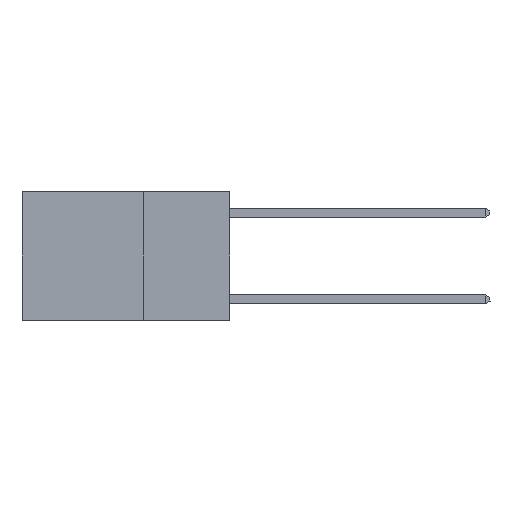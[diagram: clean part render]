
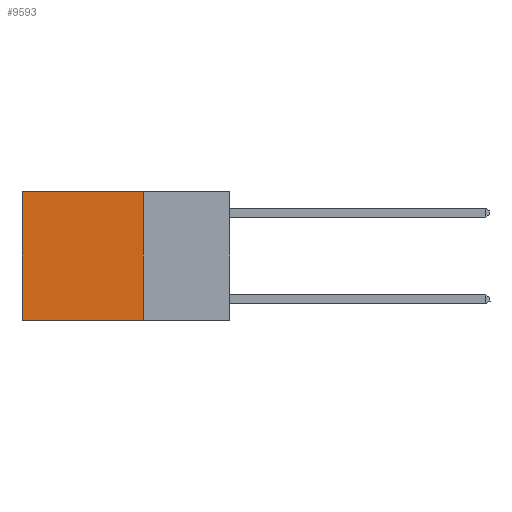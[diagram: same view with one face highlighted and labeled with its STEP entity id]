
A CAD part, left-side view. The second image highlights one B-rep face of the part: STEP entity #9593.
In plain terms, the highlighted planar face has unit normal (-1, 0, 0).
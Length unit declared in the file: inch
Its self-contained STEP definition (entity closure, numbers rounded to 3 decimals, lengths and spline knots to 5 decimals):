
#112 = DIRECTION ( 'NONE',  ( 0., 1., 0. ) ) ;
#204 = CARTESIAN_POINT ( 'NONE',  ( 0.2625, 0.25, -0.37 ) ) ;
#878 = ORIENTED_EDGE ( 'NONE', *, *, #11214, .F. ) ;
#1173 = PLANE ( 'NONE',  #4843 ) ;
#1313 = EDGE_CURVE ( 'NONE', #6642, #8136, #4791, .T. ) ;
#1764 = CARTESIAN_POINT ( 'NONE',  ( 0.2625, 0.25, 0. ) ) ;
#1929 = LINE ( 'NONE', #8316, #9382 ) ;
#2054 = VECTOR ( 'NONE', #9481, 39.37008 ) ;
#2220 = DIRECTION ( 'NONE',  ( 1., 0., 0. ) ) ;
#2715 = VERTEX_POINT ( 'NONE', #5784 ) ;
#3554 = CARTESIAN_POINT ( 'NONE',  ( 0.2625, 0.25, 0. ) ) ;
#4174 = VERTEX_POINT ( 'NONE', #204 ) ;
#4241 = CARTESIAN_POINT ( 'NONE',  ( 0.2625, 0.25, 0. ) ) ;
#4490 = CARTESIAN_POINT ( 'NONE',  ( 0.2625, 0.6, 0. ) ) ;
#4791 = LINE ( 'NONE', #10523, #2054 ) ;
#4843 = AXIS2_PLACEMENT_3D ( 'NONE', #4241, #2220, #9292 ) ;
#5443 = LINE ( 'NONE', #4490, #12897 ) ;
#5534 = DIRECTION ( 'NONE',  ( 0., 0., -1. ) ) ;
#5784 = CARTESIAN_POINT ( 'NONE',  ( 0.2625, 0.6, -0.37 ) ) ;
#5880 = VECTOR ( 'NONE', #11766, 39.37008 ) ;
#6181 = EDGE_LOOP ( 'NONE', ( #7846, #6846, #878, #9251 ) ) ;
#6642 = VERTEX_POINT ( 'NONE', #3554 ) ;
#6846 = ORIENTED_EDGE ( 'NONE', *, *, #7033, .F. ) ;
#7033 = EDGE_CURVE ( 'NONE', #4174, #2715, #1929, .T. ) ;
#7846 = ORIENTED_EDGE ( 'NONE', *, *, #9722, .T. ) ;
#8136 = VERTEX_POINT ( 'NONE', #10039 ) ;
#8316 = CARTESIAN_POINT ( 'NONE',  ( 0.2625, 0.25, -0.37 ) ) ;
#8550 = LINE ( 'NONE', #1764, #5880 ) ;
#9251 = ORIENTED_EDGE ( 'NONE', *, *, #1313, .T. ) ;
#9292 = DIRECTION ( 'NONE',  ( 0., 0., -1. ) ) ;
#9382 = VECTOR ( 'NONE', #112, 39.37008 ) ;
#9481 = DIRECTION ( 'NONE',  ( 0., 1., 0. ) ) ;
#9593 = ADVANCED_FACE ( 'NONE', ( #9797 ), #1173, .F. ) ;
#9722 = EDGE_CURVE ( 'NONE', #8136, #2715, #5443, .T. ) ;
#9797 = FACE_OUTER_BOUND ( 'NONE', #6181, .T. ) ;
#10039 = CARTESIAN_POINT ( 'NONE',  ( 0.2625, 0.6, 0. ) ) ;
#10523 = CARTESIAN_POINT ( 'NONE',  ( 0.2625, 0.25, 0. ) ) ;
#11214 = EDGE_CURVE ( 'NONE', #6642, #4174, #8550, .T. ) ;
#11766 = DIRECTION ( 'NONE',  ( 0., 0., -1. ) ) ;
#12897 = VECTOR ( 'NONE', #5534, 39.37008 ) ;
